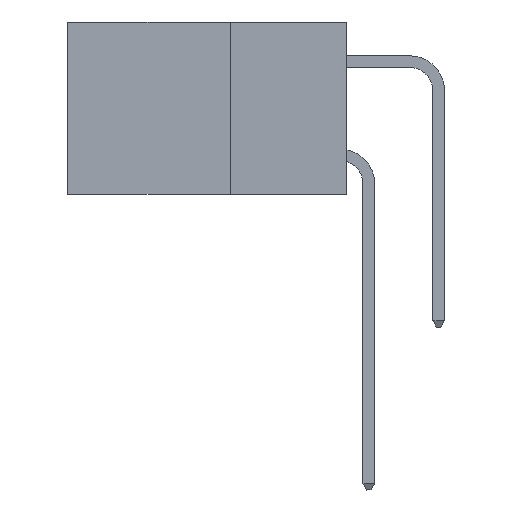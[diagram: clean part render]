
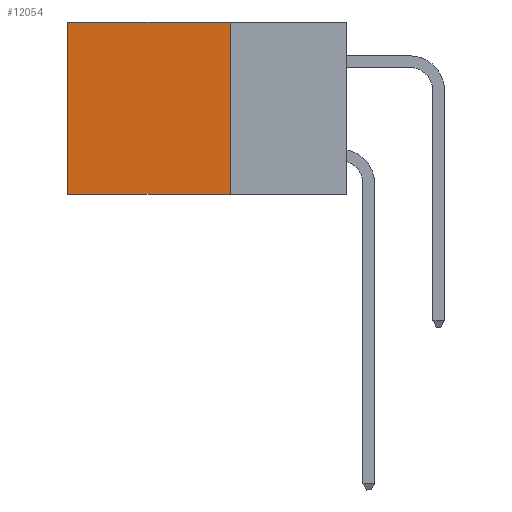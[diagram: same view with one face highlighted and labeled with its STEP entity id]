
A CAD part, left-side view. The second image highlights one B-rep face of the part: STEP entity #12054.
In plain terms, the highlighted planar face has unit normal (-1, 0, 0).
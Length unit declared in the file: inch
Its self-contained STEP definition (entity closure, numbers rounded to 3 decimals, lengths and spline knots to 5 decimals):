
#208 = CARTESIAN_POINT ( 'NONE',  ( 0.2875, 0.25, 0. ) ) ;
#280 = LINE ( 'NONE', #15243, #1170 ) ;
#288 = DIRECTION ( 'NONE',  ( 0., 0., -1. ) ) ;
#1170 = VECTOR ( 'NONE', #17046, 39.37008 ) ;
#2210 = FACE_OUTER_BOUND ( 'NONE', #21446, .T. ) ;
#2685 = CARTESIAN_POINT ( 'NONE',  ( 0.2875, 0.25, -0.37 ) ) ;
#4067 = VERTEX_POINT ( 'NONE', #13777 ) ;
#5559 = VECTOR ( 'NONE', #18877, 39.37008 ) ;
#5778 = EDGE_CURVE ( 'NONE', #4067, #17217, #8675, .T. ) ;
#6004 = DIRECTION ( 'NONE',  ( 1., 0., 0. ) ) ;
#7537 = AXIS2_PLACEMENT_3D ( 'NONE', #16938, #6004, #16688 ) ;
#8270 = VECTOR ( 'NONE', #288, 39.37008 ) ;
#8317 = EDGE_CURVE ( 'NONE', #15143, #11361, #8843, .T. ) ;
#8415 = VECTOR ( 'NONE', #18080, 39.37008 ) ;
#8675 = LINE ( 'NONE', #12641, #8415 ) ;
#8843 = LINE ( 'NONE', #208, #8270 ) ;
#9435 = PLANE ( 'NONE',  #7537 ) ;
#9585 = CARTESIAN_POINT ( 'NONE',  ( 0.2875, 0.25, -0.37 ) ) ;
#10740 = ORIENTED_EDGE ( 'NONE', *, *, #8317, .F. ) ;
#11361 = VERTEX_POINT ( 'NONE', #2685 ) ;
#11750 = CARTESIAN_POINT ( 'NONE',  ( 0.2875, 0.6, -0.37 ) ) ;
#12054 = ADVANCED_FACE ( 'NONE', ( #2210 ), #9435, .F. ) ;
#12641 = CARTESIAN_POINT ( 'NONE',  ( 0.2875, 0.6, 0. ) ) ;
#13777 = CARTESIAN_POINT ( 'NONE',  ( 0.2875, 0.6, 0. ) ) ;
#14873 = ORIENTED_EDGE ( 'NONE', *, *, #5778, .T. ) ;
#15143 = VERTEX_POINT ( 'NONE', #16392 ) ;
#15243 = CARTESIAN_POINT ( 'NONE',  ( 0.2875, 0.25, 0. ) ) ;
#16392 = CARTESIAN_POINT ( 'NONE',  ( 0.2875, 0.25, 0. ) ) ;
#16688 = DIRECTION ( 'NONE',  ( 0., 0., -1. ) ) ;
#16938 = CARTESIAN_POINT ( 'NONE',  ( 0.2875, 0.25, 0. ) ) ;
#17046 = DIRECTION ( 'NONE',  ( 0., 1., 0. ) ) ;
#17217 = VERTEX_POINT ( 'NONE', #11750 ) ;
#18080 = DIRECTION ( 'NONE',  ( 0., 0., -1. ) ) ;
#18404 = EDGE_CURVE ( 'NONE', #15143, #4067, #280, .T. ) ;
#18877 = DIRECTION ( 'NONE',  ( 0., 1., 0. ) ) ;
#19983 = LINE ( 'NONE', #9585, #5559 ) ;
#21148 = EDGE_CURVE ( 'NONE', #11361, #17217, #19983, .T. ) ;
#21446 = EDGE_LOOP ( 'NONE', ( #14873, #22677, #10740, #22518 ) ) ;
#22518 = ORIENTED_EDGE ( 'NONE', *, *, #18404, .T. ) ;
#22677 = ORIENTED_EDGE ( 'NONE', *, *, #21148, .F. ) ;
